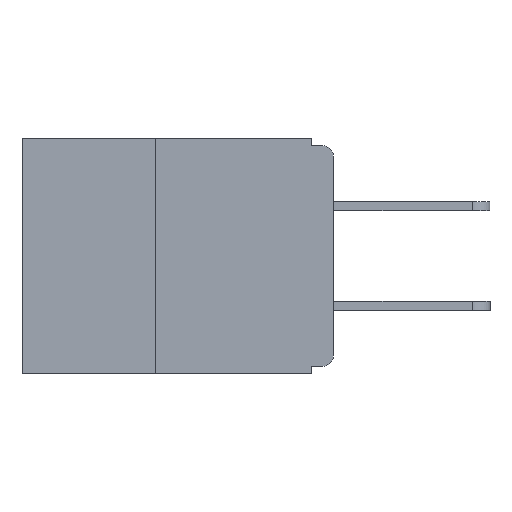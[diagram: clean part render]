
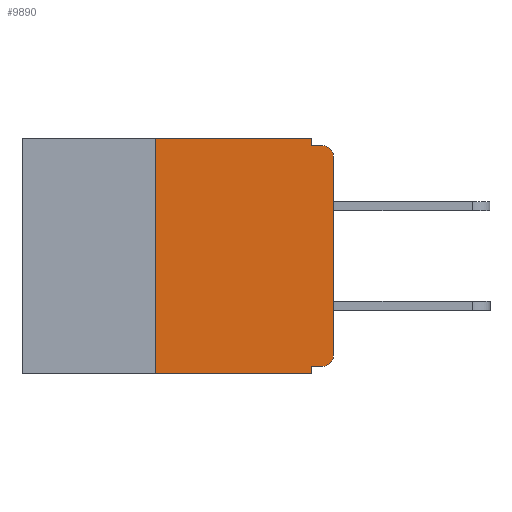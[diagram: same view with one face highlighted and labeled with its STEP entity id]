
A CAD part, left-side view. The second image highlights one B-rep face of the part: STEP entity #9890.
In plain terms, the highlighted planar face has unit normal (-1, 0, 0).
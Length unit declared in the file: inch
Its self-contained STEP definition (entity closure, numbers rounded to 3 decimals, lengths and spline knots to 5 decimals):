
#2 = LINE ( 'NONE', #8916, #1999 ) ;
#117 = DIRECTION ( 'NONE',  ( 0., 0., -1. ) ) ;
#264 = EDGE_CURVE ( 'NONE', #2213, #1673, #2411, .T. ) ;
#310 = LINE ( 'NONE', #8634, #2295 ) ;
#378 = EDGE_CURVE ( 'NONE', #9823, #3092, #9983, .T. ) ;
#460 = CARTESIAN_POINT ( 'NONE',  ( 0., 0., -0.305 ) ) ;
#527 = CARTESIAN_POINT ( 'NONE',  ( 0., 0.031, 0. ) ) ;
#1168 = ORIENTED_EDGE ( 'NONE', *, *, #5785, .T. ) ;
#1261 = FACE_OUTER_BOUND ( 'NONE', #4710, .T. ) ;
#1386 = CARTESIAN_POINT ( 'NONE',  ( 0., 0., 0. ) ) ;
#1394 = EDGE_CURVE ( 'NONE', #1673, #2467, #2, .T. ) ;
#1440 = CARTESIAN_POINT ( 'NONE',  ( 0., 0.25, -0.33 ) ) ;
#1673 = VERTEX_POINT ( 'NONE', #3306 ) ;
#1700 = DIRECTION ( 'NONE',  ( 0., 0., -1. ) ) ;
#1850 = CIRCLE ( 'NONE', #1889, 0.015 ) ;
#1874 = DIRECTION ( 'NONE',  ( 0., 0., -1. ) ) ;
#1889 = AXIS2_PLACEMENT_3D ( 'NONE', #3480, #10292, #1874 ) ;
#1999 = VECTOR ( 'NONE', #6192, 39.37008 ) ;
#2213 = VERTEX_POINT ( 'NONE', #2571 ) ;
#2295 = VECTOR ( 'NONE', #9472, 39.37008 ) ;
#2411 = LINE ( 'NONE', #6659, #8802 ) ;
#2443 = DIRECTION ( 'NONE',  ( 0., 1., 0. ) ) ;
#2462 = ORIENTED_EDGE ( 'NONE', *, *, #378, .F. ) ;
#2467 = VERTEX_POINT ( 'NONE', #7114 ) ;
#2548 = VERTEX_POINT ( 'NONE', #2897 ) ;
#2571 = CARTESIAN_POINT ( 'NONE',  ( 0., 0.015, -0.32 ) ) ;
#2597 = CARTESIAN_POINT ( 'NONE',  ( 0., 0.25, -0.33 ) ) ;
#2640 = CARTESIAN_POINT ( 'NONE',  ( 0., 0., -0.01 ) ) ;
#2862 = EDGE_CURVE ( 'NONE', #10624, #2548, #1850, .T. ) ;
#2897 = CARTESIAN_POINT ( 'NONE',  ( 0., 0.015, -0.01 ) ) ;
#3052 = LINE ( 'NONE', #9419, #6873 ) ;
#3092 = VERTEX_POINT ( 'NONE', #6472 ) ;
#3306 = CARTESIAN_POINT ( 'NONE',  ( 0., 0.031, -0.32 ) ) ;
#3392 = CARTESIAN_POINT ( 'NONE',  ( 0., 0.437, 0. ) ) ;
#3438 = EDGE_CURVE ( 'NONE', #10794, #5557, #3052, .T. ) ;
#3439 = CARTESIAN_POINT ( 'NONE',  ( 0., 0., -0.025 ) ) ;
#3480 = CARTESIAN_POINT ( 'NONE',  ( 0., 0.015, -0.025 ) ) ;
#3546 = DIRECTION ( 'NONE',  ( 0., 0., -1. ) ) ;
#3986 = VERTEX_POINT ( 'NONE', #460 ) ;
#4024 = ORIENTED_EDGE ( 'NONE', *, *, #4136, .F. ) ;
#4089 = ORIENTED_EDGE ( 'NONE', *, *, #3438, .F. ) ;
#4136 = EDGE_CURVE ( 'NONE', #5557, #2548, #5656, .T. ) ;
#4186 = EDGE_CURVE ( 'NONE', #2213, #3986, #8724, .T. ) ;
#4710 = EDGE_LOOP ( 'NONE', ( #1168, #9516, #4024, #4089, #5441, #2462, #10601, #10864, #5919, #6904 ) ) ;
#5104 = VECTOR ( 'NONE', #9165, 39.37008 ) ;
#5369 = LINE ( 'NONE', #8165, #9877 ) ;
#5441 = ORIENTED_EDGE ( 'NONE', *, *, #10215, .F. ) ;
#5557 = VERTEX_POINT ( 'NONE', #9061 ) ;
#5656 = LINE ( 'NONE', #2640, #10430 ) ;
#5785 = EDGE_CURVE ( 'NONE', #3986, #10624, #8166, .T. ) ;
#5919 = ORIENTED_EDGE ( 'NONE', *, *, #264, .F. ) ;
#6192 = DIRECTION ( 'NONE',  ( 0., 0., -1. ) ) ;
#6420 = DIRECTION ( 'NONE',  ( 0., -1., 0. ) ) ;
#6472 = CARTESIAN_POINT ( 'NONE',  ( 0., 0.25, 0. ) ) ;
#6659 = CARTESIAN_POINT ( 'NONE',  ( 0., 0., -0.32 ) ) ;
#6665 = DIRECTION ( 'NONE',  ( 1., 0., 0. ) ) ;
#6820 = PLANE ( 'NONE',  #8704 ) ;
#6873 = VECTOR ( 'NONE', #117, 39.37008 ) ;
#6904 = ORIENTED_EDGE ( 'NONE', *, *, #4186, .T. ) ;
#7114 = CARTESIAN_POINT ( 'NONE',  ( 0., 0.031, -0.33 ) ) ;
#7285 = AXIS2_PLACEMENT_3D ( 'NONE', #7753, #8696, #3546 ) ;
#7753 = CARTESIAN_POINT ( 'NONE',  ( 0., 0.015, -0.305 ) ) ;
#8165 = CARTESIAN_POINT ( 'NONE',  ( 0., 0.437, -0.33 ) ) ;
#8166 = LINE ( 'NONE', #1386, #5104 ) ;
#8427 = EDGE_CURVE ( 'NONE', #9823, #2467, #5369, .T. ) ;
#8634 = CARTESIAN_POINT ( 'NONE',  ( 0., 0.437, 0. ) ) ;
#8696 = DIRECTION ( 'NONE',  ( -1., 0., 0. ) ) ;
#8704 = AXIS2_PLACEMENT_3D ( 'NONE', #3392, #6665, #1700 ) ;
#8724 = CIRCLE ( 'NONE', #7285, 0.015 ) ;
#8802 = VECTOR ( 'NONE', #2443, 39.37008 ) ;
#8916 = CARTESIAN_POINT ( 'NONE',  ( 0., 0.031, -0.33 ) ) ;
#9061 = CARTESIAN_POINT ( 'NONE',  ( 0., 0.031, -0.01 ) ) ;
#9165 = DIRECTION ( 'NONE',  ( 0., 0., 1. ) ) ;
#9417 = DIRECTION ( 'NONE',  ( 0., 0., 1. ) ) ;
#9419 = CARTESIAN_POINT ( 'NONE',  ( 0., 0.031, 0. ) ) ;
#9421 = DIRECTION ( 'NONE',  ( 0., -1., 0. ) ) ;
#9472 = DIRECTION ( 'NONE',  ( 0., -1., 0. ) ) ;
#9516 = ORIENTED_EDGE ( 'NONE', *, *, #2862, .T. ) ;
#9823 = VERTEX_POINT ( 'NONE', #1440 ) ;
#9877 = VECTOR ( 'NONE', #6420, 39.37008 ) ;
#9890 = ADVANCED_FACE ( 'NONE', ( #1261 ), #6820, .F. ) ;
#9983 = LINE ( 'NONE', #2597, #10912 ) ;
#10215 = EDGE_CURVE ( 'NONE', #3092, #10794, #310, .T. ) ;
#10292 = DIRECTION ( 'NONE',  ( -1., 0., 0. ) ) ;
#10430 = VECTOR ( 'NONE', #9421, 39.37008 ) ;
#10601 = ORIENTED_EDGE ( 'NONE', *, *, #8427, .T. ) ;
#10624 = VERTEX_POINT ( 'NONE', #3439 ) ;
#10794 = VERTEX_POINT ( 'NONE', #527 ) ;
#10864 = ORIENTED_EDGE ( 'NONE', *, *, #1394, .F. ) ;
#10912 = VECTOR ( 'NONE', #9417, 39.37008 ) ;
